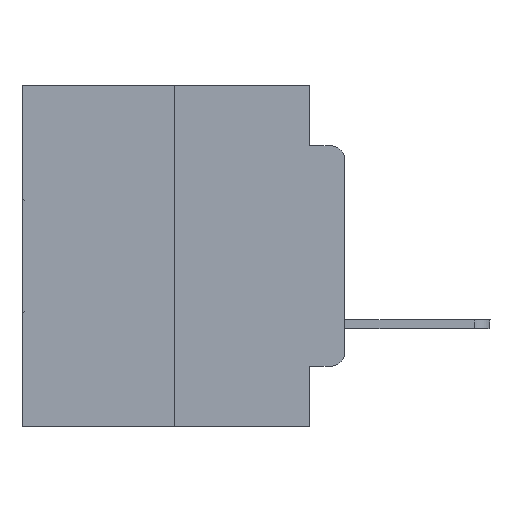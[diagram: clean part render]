
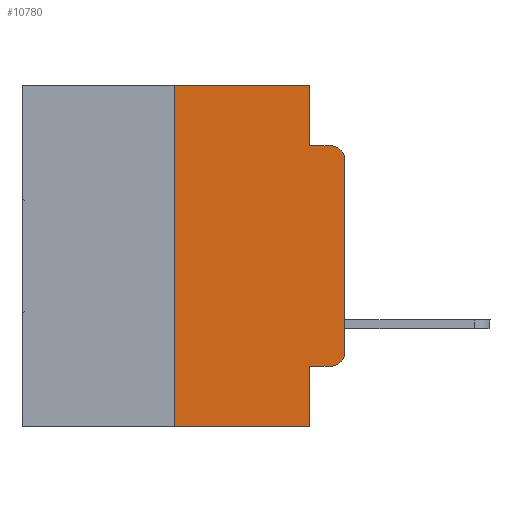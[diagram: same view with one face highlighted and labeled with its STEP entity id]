
A CAD part, left-side view. The second image highlights one B-rep face of the part: STEP entity #10780.
In plain terms, the highlighted planar face has unit normal (-1, 0, 0).
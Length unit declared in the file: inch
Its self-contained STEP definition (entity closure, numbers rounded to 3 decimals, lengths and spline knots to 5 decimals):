
#71 = LINE ( 'NONE', #20466, #13874 ) ;
#399 = ORIENTED_EDGE ( 'NONE', *, *, #5406, .F. ) ;
#919 = CIRCLE ( 'NONE', #2380, 0.02 ) ;
#963 = VECTOR ( 'NONE', #19050, 39.37008 ) ;
#1002 = LINE ( 'NONE', #9770, #21909 ) ;
#1150 = DIRECTION ( 'NONE',  ( 0., 0., -1. ) ) ;
#1360 = AXIS2_PLACEMENT_3D ( 'NONE', #3055, #8020, #12422 ) ;
#1615 = ORIENTED_EDGE ( 'NONE', *, *, #27630, .F. ) ;
#1931 = DIRECTION ( 'NONE',  ( 0., -1., 0. ) ) ;
#1983 = DIRECTION ( 'NONE',  ( 0., 0., 1. ) ) ;
#2380 = AXIS2_PLACEMENT_3D ( 'NONE', #24082, #28466, #14310 ) ;
#2999 = CARTESIAN_POINT ( 'NONE',  ( 0., 0.25, 0. ) ) ;
#3055 = CARTESIAN_POINT ( 'NONE',  ( 0., 0.473, 0. ) ) ;
#3678 = VERTEX_POINT ( 'NONE', #2999 ) ;
#3766 = EDGE_CURVE ( 'NONE', #29777, #10964, #5415, .T. ) ;
#4420 = CARTESIAN_POINT ( 'NONE',  ( 0., 0.02, -0.0885 ) ) ;
#4724 = ORIENTED_EDGE ( 'NONE', *, *, #26081, .T. ) ;
#5406 = EDGE_CURVE ( 'NONE', #10137, #10964, #1002, .T. ) ;
#5415 = LINE ( 'NONE', #8109, #14775 ) ;
#5531 = CIRCLE ( 'NONE', #11826, 0.02 ) ;
#5860 = VERTEX_POINT ( 'NONE', #26330 ) ;
#7884 = CARTESIAN_POINT ( 'NONE',  ( 0., 0., -0.3915 ) ) ;
#7911 = CARTESIAN_POINT ( 'NONE',  ( 0., 0.25, -0.5 ) ) ;
#8020 = DIRECTION ( 'NONE',  ( 1., 0., 0. ) ) ;
#8109 = CARTESIAN_POINT ( 'NONE',  ( 0., 0.473, -0.5 ) ) ;
#8376 = ORIENTED_EDGE ( 'NONE', *, *, #12091, .T. ) ;
#8465 = CARTESIAN_POINT ( 'NONE',  ( 0., 0.051, -0.5 ) ) ;
#8969 = LINE ( 'NONE', #18210, #15307 ) ;
#9432 = DIRECTION ( 'NONE',  ( -1., 0., 0. ) ) ;
#9713 = VECTOR ( 'NONE', #24496, 39.37008 ) ;
#9744 = EDGE_CURVE ( 'NONE', #10137, #26079, #71, .T. ) ;
#9770 = CARTESIAN_POINT ( 'NONE',  ( 0., 0.051, 0. ) ) ;
#9842 = EDGE_CURVE ( 'NONE', #3678, #5860, #8969, .T. ) ;
#10137 = VERTEX_POINT ( 'NONE', #24635 ) ;
#10780 = ADVANCED_FACE ( 'NONE', ( #16974 ), #14689, .F. ) ;
#10964 = VERTEX_POINT ( 'NONE', #8465 ) ;
#11408 = ORIENTED_EDGE ( 'NONE', *, *, #17504, .T. ) ;
#11658 = ORIENTED_EDGE ( 'NONE', *, *, #13771, .F. ) ;
#11826 = AXIS2_PLACEMENT_3D ( 'NONE', #20914, #9432, #21507 ) ;
#12091 = EDGE_CURVE ( 'NONE', #13423, #23913, #29452, .T. ) ;
#12422 = DIRECTION ( 'NONE',  ( 0., 0., -1. ) ) ;
#12976 = CARTESIAN_POINT ( 'NONE',  ( 0., 0.051, -0.0885 ) ) ;
#13147 = VERTEX_POINT ( 'NONE', #26971 ) ;
#13347 = EDGE_LOOP ( 'NONE', ( #8376, #11408, #1615, #11658, #25595, #23353, #25678, #399, #15032, #4724 ) ) ;
#13423 = VERTEX_POINT ( 'NONE', #7884 ) ;
#13771 = EDGE_CURVE ( 'NONE', #5860, #13147, #26568, .T. ) ;
#13874 = VECTOR ( 'NONE', #20605, 39.37008 ) ;
#14310 = DIRECTION ( 'NONE',  ( 0., 0., -1. ) ) ;
#14689 = PLANE ( 'NONE',  #1360 ) ;
#14775 = VECTOR ( 'NONE', #1931, 39.37008 ) ;
#15032 = ORIENTED_EDGE ( 'NONE', *, *, #9744, .T. ) ;
#15276 = VECTOR ( 'NONE', #19468, 39.37008 ) ;
#15307 = VECTOR ( 'NONE', #27385, 39.37008 ) ;
#16931 = LINE ( 'NONE', #12976, #15276 ) ;
#16974 = FACE_OUTER_BOUND ( 'NONE', #13347, .T. ) ;
#17504 = EDGE_CURVE ( 'NONE', #23913, #25186, #919, .T. ) ;
#17739 = CARTESIAN_POINT ( 'NONE',  ( 0., 0.25, 0. ) ) ;
#18210 = CARTESIAN_POINT ( 'NONE',  ( 0., 0.473, 0. ) ) ;
#18288 = CARTESIAN_POINT ( 'NONE',  ( 0., 0., -0.1085 ) ) ;
#19050 = DIRECTION ( 'NONE',  ( 0., 0., -1. ) ) ;
#19468 = DIRECTION ( 'NONE',  ( 0., -1., 0. ) ) ;
#19488 = CARTESIAN_POINT ( 'NONE',  ( 0., 0.051, 0. ) ) ;
#20466 = CARTESIAN_POINT ( 'NONE',  ( 0., 0.051, -0.4115 ) ) ;
#20605 = DIRECTION ( 'NONE',  ( 0., -1., 0. ) ) ;
#20914 = CARTESIAN_POINT ( 'NONE',  ( 0., 0.02, -0.3915 ) ) ;
#21507 = DIRECTION ( 'NONE',  ( 0., 0., -1. ) ) ;
#21909 = VECTOR ( 'NONE', #1150, 39.37008 ) ;
#23144 = VECTOR ( 'NONE', #1983, 39.37008 ) ;
#23353 = ORIENTED_EDGE ( 'NONE', *, *, #28604, .F. ) ;
#23913 = VERTEX_POINT ( 'NONE', #18288 ) ;
#24082 = CARTESIAN_POINT ( 'NONE',  ( 0., 0.02, -0.1085 ) ) ;
#24496 = DIRECTION ( 'NONE',  ( 0., 0., 1. ) ) ;
#24635 = CARTESIAN_POINT ( 'NONE',  ( 0., 0.051, -0.4115 ) ) ;
#25186 = VERTEX_POINT ( 'NONE', #4420 ) ;
#25595 = ORIENTED_EDGE ( 'NONE', *, *, #9842, .F. ) ;
#25678 = ORIENTED_EDGE ( 'NONE', *, *, #3766, .T. ) ;
#26079 = VERTEX_POINT ( 'NONE', #28003 ) ;
#26081 = EDGE_CURVE ( 'NONE', #26079, #13423, #5531, .T. ) ;
#26330 = CARTESIAN_POINT ( 'NONE',  ( 0., 0.051, 0. ) ) ;
#26568 = LINE ( 'NONE', #19488, #963 ) ;
#26781 = LINE ( 'NONE', #17739, #9713 ) ;
#26894 = CARTESIAN_POINT ( 'NONE',  ( 0., 0., 0. ) ) ;
#26971 = CARTESIAN_POINT ( 'NONE',  ( 0., 0.051, -0.0885 ) ) ;
#27385 = DIRECTION ( 'NONE',  ( 0., -1., 0. ) ) ;
#27630 = EDGE_CURVE ( 'NONE', #13147, #25186, #16931, .T. ) ;
#28003 = CARTESIAN_POINT ( 'NONE',  ( 0., 0.02, -0.4115 ) ) ;
#28466 = DIRECTION ( 'NONE',  ( -1., 0., 0. ) ) ;
#28604 = EDGE_CURVE ( 'NONE', #29777, #3678, #26781, .T. ) ;
#29452 = LINE ( 'NONE', #26894, #23144 ) ;
#29777 = VERTEX_POINT ( 'NONE', #7911 ) ;
